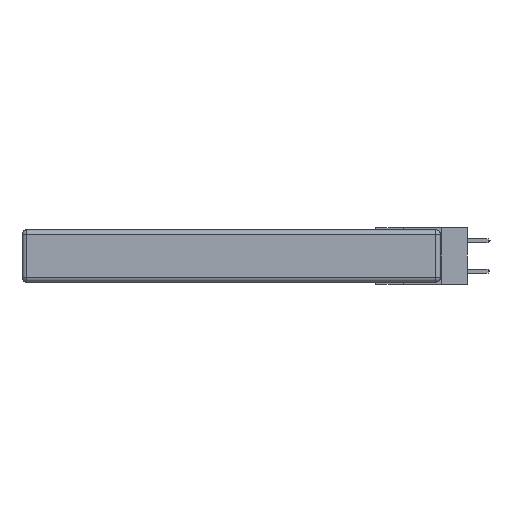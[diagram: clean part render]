
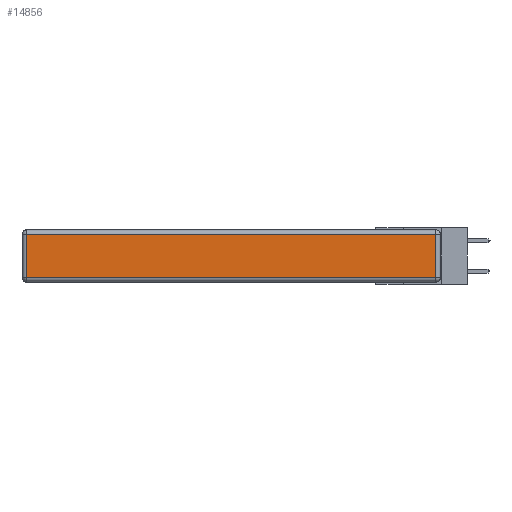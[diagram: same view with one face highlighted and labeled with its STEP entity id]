
A CAD part, left-side view. The second image highlights one B-rep face of the part: STEP entity #14856.
In plain terms, the highlighted planar face has unit normal (-1, 0, 0).
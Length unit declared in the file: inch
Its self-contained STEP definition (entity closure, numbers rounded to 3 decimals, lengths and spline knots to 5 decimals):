
#1988 = CARTESIAN_POINT ( 'NONE',  ( 0., 0.03, -0.313 ) ) ;
#4147 = VERTEX_POINT ( 'NONE', #18283 ) ;
#4616 = DIRECTION ( 'NONE',  ( 0., 0., -1. ) ) ;
#4660 = PLANE ( 'NONE',  #20157 ) ;
#6015 = DIRECTION ( 'NONE',  ( -1., 0., 0. ) ) ;
#6897 = VERTEX_POINT ( 'NONE', #12797 ) ;
#8380 = ORIENTED_EDGE ( 'NONE', *, *, #12376, .T. ) ;
#8741 = LINE ( 'NONE', #11345, #12320 ) ;
#9481 = DIRECTION ( 'NONE',  ( 0., 1., 0. ) ) ;
#10250 = FACE_OUTER_BOUND ( 'NONE', #12030, .T. ) ;
#11345 = CARTESIAN_POINT ( 'NONE',  ( 0., 0., -0.313 ) ) ;
#12030 = EDGE_LOOP ( 'NONE', ( #18375, #23182, #8380, #15737 ) ) ;
#12320 = VECTOR ( 'NONE', #15237, 39.37008 ) ;
#12328 = LINE ( 'NONE', #12954, #26134 ) ;
#12376 = EDGE_CURVE ( 'NONE', #4147, #6897, #23143, .T. ) ;
#12797 = CARTESIAN_POINT ( 'NONE',  ( 0., 2.72, -0.03 ) ) ;
#12954 = CARTESIAN_POINT ( 'NONE',  ( 0., 2.72, -0.343 ) ) ;
#14115 = VECTOR ( 'NONE', #16830, 39.37008 ) ;
#14627 = CARTESIAN_POINT ( 'NONE',  ( 0., 0.03, -0.343 ) ) ;
#14856 = ADVANCED_FACE ( 'NONE', ( #10250 ), #4660, .T. ) ;
#15237 = DIRECTION ( 'NONE',  ( 0., -1., 0. ) ) ;
#15737 = ORIENTED_EDGE ( 'NONE', *, *, #21418, .T. ) ;
#16507 = DIRECTION ( 'NONE',  ( 0., 0., 1. ) ) ;
#16830 = DIRECTION ( 'NONE',  ( 0., 0., 1. ) ) ;
#17640 = VECTOR ( 'NONE', #9481, 39.37008 ) ;
#17913 = CARTESIAN_POINT ( 'NONE',  ( 0., 2.75, -0.03 ) ) ;
#18283 = CARTESIAN_POINT ( 'NONE',  ( 0., 0.03, -0.03 ) ) ;
#18375 = ORIENTED_EDGE ( 'NONE', *, *, #18782, .T. ) ;
#18489 = CARTESIAN_POINT ( 'NONE',  ( 0., 2.72, -0.313 ) ) ;
#18525 = VERTEX_POINT ( 'NONE', #1988 ) ;
#18782 = EDGE_CURVE ( 'NONE', #23957, #18525, #8741, .T. ) ;
#19665 = LINE ( 'NONE', #14627, #14115 ) ;
#20157 = AXIS2_PLACEMENT_3D ( 'NONE', #25578, #6015, #16507 ) ;
#21418 = EDGE_CURVE ( 'NONE', #6897, #23957, #12328, .T. ) ;
#23143 = LINE ( 'NONE', #17913, #17640 ) ;
#23182 = ORIENTED_EDGE ( 'NONE', *, *, #25660, .T. ) ;
#23957 = VERTEX_POINT ( 'NONE', #18489 ) ;
#25578 = CARTESIAN_POINT ( 'NONE',  ( 0., 0., -0.343 ) ) ;
#25660 = EDGE_CURVE ( 'NONE', #18525, #4147, #19665, .T. ) ;
#26134 = VECTOR ( 'NONE', #4616, 39.37008 ) ;
